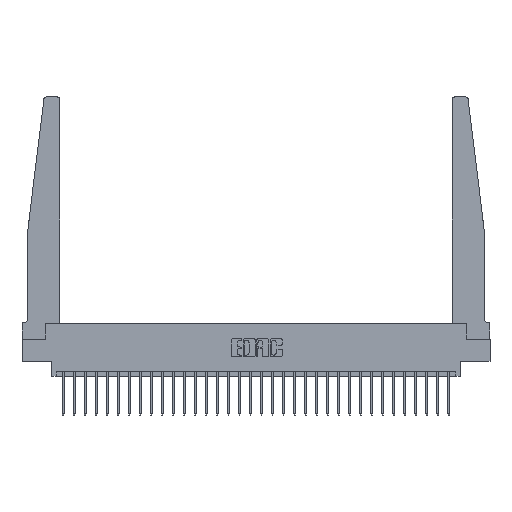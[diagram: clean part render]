
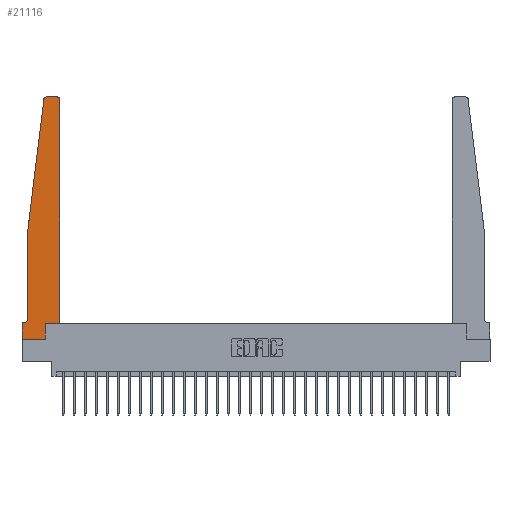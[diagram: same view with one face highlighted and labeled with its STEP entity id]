
A CAD part, top view. The second image highlights one B-rep face of the part: STEP entity #21116.
In plain terms, the highlighted planar face has unit normal (0, 0, 1).
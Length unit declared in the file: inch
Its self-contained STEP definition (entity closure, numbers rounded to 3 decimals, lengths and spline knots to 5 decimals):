
#177 = VERTEX_POINT ( 'NONE', #24641 ) ;
#543 = CARTESIAN_POINT ( 'NONE',  ( 0.2605, 0.18, 0.37 ) ) ;
#710 = VECTOR ( 'NONE', #4075, 39.37008 ) ;
#756 = CARTESIAN_POINT ( 'NONE',  ( 0.015, 0.2375, 0.37 ) ) ;
#824 = EDGE_CURVE ( 'NONE', #18573, #177, #5502, .T. ) ;
#1322 = DIRECTION ( 'NONE',  ( 0., 0., 1. ) ) ;
#1462 = CARTESIAN_POINT ( 'NONE',  ( 0., 0., 0.37 ) ) ;
#1492 = DIRECTION ( 'NONE',  ( 1., 0., 0. ) ) ;
#1540 = ORIENTED_EDGE ( 'NONE', *, *, #13377, .T. ) ;
#1813 = VERTEX_POINT ( 'NONE', #18980 ) ;
#1875 = VECTOR ( 'NONE', #4277, 39.37008 ) ;
#1993 = CARTESIAN_POINT ( 'NONE',  ( 0.25, 2.75, 0.37 ) ) ;
#2558 = ORIENTED_EDGE ( 'NONE', *, *, #5002, .T. ) ;
#2577 = ORIENTED_EDGE ( 'NONE', *, *, #8632, .T. ) ;
#2834 = EDGE_CURVE ( 'NONE', #1813, #8471, #23170, .T. ) ;
#3036 = DIRECTION ( 'NONE',  ( -1., 0., 0. ) ) ;
#3135 = CIRCLE ( 'NONE', #17296, 0.03 ) ;
#3824 = DIRECTION ( 'NONE',  ( 1., 0., 0. ) ) ;
#3837 = EDGE_CURVE ( 'NONE', #177, #1813, #16126, .T. ) ;
#4075 = DIRECTION ( 'NONE',  ( 1., 0., 0. ) ) ;
#4108 = VECTOR ( 'NONE', #6024, 39.37008 ) ;
#4277 = DIRECTION ( 'NONE',  ( -1., 0., 0. ) ) ;
#4627 = DIRECTION ( 'NONE',  ( 0., 0., 1. ) ) ;
#4763 = VECTOR ( 'NONE', #3824, 39.37008 ) ;
#4905 = ORIENTED_EDGE ( 'NONE', *, *, #22280, .T. ) ;
#4918 = CARTESIAN_POINT ( 'NONE',  ( 0.065, 0.1875, 0.37 ) ) ;
#5002 = EDGE_CURVE ( 'NONE', #22477, #9192, #5044, .T. ) ;
#5044 = LINE ( 'NONE', #14678, #22388 ) ;
#5111 = DIRECTION ( 'NONE',  ( 0., 1., 0. ) ) ;
#5195 = CARTESIAN_POINT ( 'NONE',  ( 0.065, 0.2375, 0.37 ) ) ;
#5502 = LINE ( 'NONE', #543, #28806 ) ;
#6024 = DIRECTION ( 'NONE',  ( 0., -1., 0. ) ) ;
#6523 = VERTEX_POINT ( 'NONE', #6734 ) ;
#6734 = CARTESIAN_POINT ( 'NONE',  ( 0.24675, 2.72367, 0.37 ) ) ;
#6892 = FACE_OUTER_BOUND ( 'NONE', #14948, .T. ) ;
#7185 = LINE ( 'NONE', #1993, #1875 ) ;
#7433 = LINE ( 'NONE', #10813, #710 ) ;
#8471 = VERTEX_POINT ( 'NONE', #27343 ) ;
#8632 = EDGE_CURVE ( 'NONE', #9192, #17447, #13394, .T. ) ;
#8838 = CARTESIAN_POINT ( 'NONE',  ( 0., 0.1875, 0.37 ) ) ;
#8934 = VERTEX_POINT ( 'NONE', #8838 ) ;
#9192 = VERTEX_POINT ( 'NONE', #5195 ) ;
#9443 = ORIENTED_EDGE ( 'NONE', *, *, #15417, .T. ) ;
#10122 = LINE ( 'NONE', #1462, #4108 ) ;
#10268 = DIRECTION ( 'NONE',  ( 0., -1., 0. ) ) ;
#10351 = PLANE ( 'NONE',  #18962 ) ;
#10361 = CARTESIAN_POINT ( 'NONE',  ( 0.2605, 0., 0.37 ) ) ;
#10487 = VERTEX_POINT ( 'NONE', #15696 ) ;
#10813 = CARTESIAN_POINT ( 'NONE',  ( 0., 0., 0.37 ) ) ;
#11226 = ORIENTED_EDGE ( 'NONE', *, *, #13471, .T. ) ;
#11250 = VECTOR ( 'NONE', #14078, 39.37008 ) ;
#11397 = AXIS2_PLACEMENT_3D ( 'NONE', #756, #16627, #3036 ) ;
#12065 = CARTESIAN_POINT ( 'NONE',  ( 0.065, 1.25, 0.37 ) ) ;
#13377 = EDGE_CURVE ( 'NONE', #28559, #6523, #15638, .T. ) ;
#13394 = CIRCLE ( 'NONE', #11397, 0.05 ) ;
#13471 = EDGE_CURVE ( 'NONE', #26703, #18573, #7433, .T. ) ;
#13939 = LINE ( 'NONE', #19339, #25903 ) ;
#14078 = DIRECTION ( 'NONE',  ( -1., 0., 0. ) ) ;
#14678 = CARTESIAN_POINT ( 'NONE',  ( 0.065, 1.25, 0.37 ) ) ;
#14940 = CARTESIAN_POINT ( 'NONE',  ( 0., 0.1875, 0.37 ) ) ;
#14948 = EDGE_LOOP ( 'NONE', ( #9443, #1540, #23719, #2558, #2577, #16279, #26381, #11226, #22134, #22343, #16089, #4905 ) ) ;
#15101 = DIRECTION ( 'NONE',  ( 0., 0., 1. ) ) ;
#15143 = CARTESIAN_POINT ( 'NONE',  ( 0.425, 0.18, 0.37 ) ) ;
#15417 = EDGE_CURVE ( 'NONE', #10487, #28559, #7185, .T. ) ;
#15638 = CIRCLE ( 'NONE', #23757, 0.03 ) ;
#15696 = CARTESIAN_POINT ( 'NONE',  ( 0.395, 2.75, 0.37 ) ) ;
#16089 = ORIENTED_EDGE ( 'NONE', *, *, #2834, .T. ) ;
#16126 = LINE ( 'NONE', #15143, #4763 ) ;
#16279 = ORIENTED_EDGE ( 'NONE', *, *, #19016, .T. ) ;
#16627 = DIRECTION ( 'NONE',  ( 0., 0., -1. ) ) ;
#17183 = DIRECTION ( 'NONE',  ( -0.122, -0.992, 0. ) ) ;
#17194 = VECTOR ( 'NONE', #20478, 39.37008 ) ;
#17209 = DIRECTION ( 'NONE',  ( 1., 0., 0. ) ) ;
#17296 = AXIS2_PLACEMENT_3D ( 'NONE', #18214, #4627, #20442 ) ;
#17447 = VERTEX_POINT ( 'NONE', #17977 ) ;
#17977 = CARTESIAN_POINT ( 'NONE',  ( 0.015, 0.1875, 0.37 ) ) ;
#18214 = CARTESIAN_POINT ( 'NONE',  ( 0.395, 2.72, 0.37 ) ) ;
#18573 = VERTEX_POINT ( 'NONE', #10361 ) ;
#18753 = CARTESIAN_POINT ( 'NONE',  ( 0., 0., 0.37 ) ) ;
#18962 = AXIS2_PLACEMENT_3D ( 'NONE', #14940, #1322, #17209 ) ;
#18980 = CARTESIAN_POINT ( 'NONE',  ( 0.425, 0.18, 0.37 ) ) ;
#19016 = EDGE_CURVE ( 'NONE', #17447, #8934, #29220, .T. ) ;
#19339 = CARTESIAN_POINT ( 'NONE',  ( 0.065, 1.25, 0.37 ) ) ;
#20386 = CARTESIAN_POINT ( 'NONE',  ( 0.425, 0.18, 0.37 ) ) ;
#20442 = DIRECTION ( 'NONE',  ( 1., 0., 0. ) ) ;
#20478 = DIRECTION ( 'NONE',  ( 0., 1., 0. ) ) ;
#20489 = EDGE_CURVE ( 'NONE', #8934, #26703, #10122, .T. ) ;
#20566 = CARTESIAN_POINT ( 'NONE',  ( 0.27653, 2.75, 0.37 ) ) ;
#21116 = ADVANCED_FACE ( 'NONE', ( #6892 ), #10351, .T. ) ;
#22134 = ORIENTED_EDGE ( 'NONE', *, *, #824, .T. ) ;
#22280 = EDGE_CURVE ( 'NONE', #8471, #10487, #3135, .T. ) ;
#22343 = ORIENTED_EDGE ( 'NONE', *, *, #3837, .T. ) ;
#22388 = VECTOR ( 'NONE', #10268, 39.37008 ) ;
#22477 = VERTEX_POINT ( 'NONE', #12065 ) ;
#23170 = LINE ( 'NONE', #20386, #17194 ) ;
#23719 = ORIENTED_EDGE ( 'NONE', *, *, #26898, .T. ) ;
#23757 = AXIS2_PLACEMENT_3D ( 'NONE', #28560, #15101, #1492 ) ;
#24641 = CARTESIAN_POINT ( 'NONE',  ( 0.2605, 0.18, 0.37 ) ) ;
#25903 = VECTOR ( 'NONE', #17183, 39.37008 ) ;
#26381 = ORIENTED_EDGE ( 'NONE', *, *, #20489, .T. ) ;
#26703 = VERTEX_POINT ( 'NONE', #18753 ) ;
#26898 = EDGE_CURVE ( 'NONE', #6523, #22477, #13939, .T. ) ;
#27343 = CARTESIAN_POINT ( 'NONE',  ( 0.425, 2.72, 0.37 ) ) ;
#28559 = VERTEX_POINT ( 'NONE', #20566 ) ;
#28560 = CARTESIAN_POINT ( 'NONE',  ( 0.27653, 2.72, 0.37 ) ) ;
#28806 = VECTOR ( 'NONE', #5111, 39.37008 ) ;
#29220 = LINE ( 'NONE', #4918, #11250 ) ;
